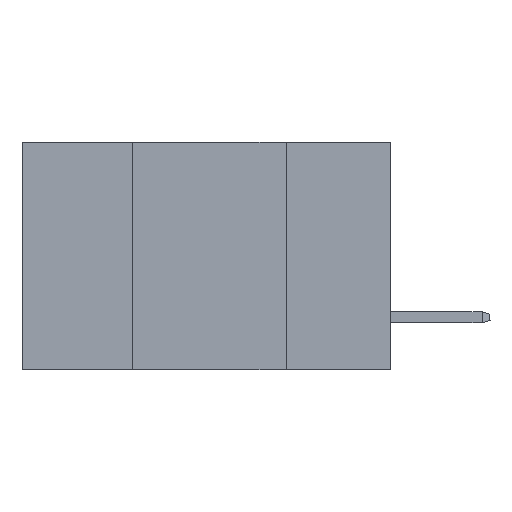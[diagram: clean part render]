
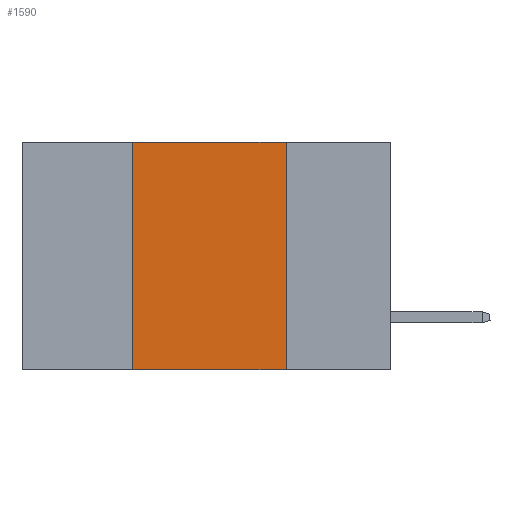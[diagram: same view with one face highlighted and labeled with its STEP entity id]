
A CAD part, left-side view. The second image highlights one B-rep face of the part: STEP entity #1590.
In plain terms, the highlighted planar face has unit normal (-1, 0, 0).
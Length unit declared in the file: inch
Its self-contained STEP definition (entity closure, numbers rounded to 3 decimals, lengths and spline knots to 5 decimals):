
#1293 = CARTESIAN_POINT ( 'NONE',  ( 0., 0.17, 0. ) ) ;
#1590 = ADVANCED_FACE ( 'NONE', ( #4072 ), #20724, .F. ) ;
#1741 = ORIENTED_EDGE ( 'NONE', *, *, #5785, .T. ) ;
#2574 = CARTESIAN_POINT ( 'NONE',  ( 0., 0.42, -0.37 ) ) ;
#3450 = CARTESIAN_POINT ( 'NONE',  ( 0., 0.6, 0. ) ) ;
#4072 = FACE_OUTER_BOUND ( 'NONE', #17372, .T. ) ;
#4275 = ORIENTED_EDGE ( 'NONE', *, *, #7892, .F. ) ;
#4960 = CARTESIAN_POINT ( 'NONE',  ( 0., 0.42, 0. ) ) ;
#5785 = EDGE_CURVE ( 'NONE', #17958, #6921, #11156, .T. ) ;
#6727 = VERTEX_POINT ( 'NONE', #1293 ) ;
#6910 = VECTOR ( 'NONE', #20247, 39.37008 ) ;
#6921 = VERTEX_POINT ( 'NONE', #15824 ) ;
#7892 = EDGE_CURVE ( 'NONE', #19741, #6727, #8213, .T. ) ;
#8213 = LINE ( 'NONE', #24294, #20574 ) ;
#9295 = DIRECTION ( 'NONE',  ( 0., 0., -1. ) ) ;
#11156 = LINE ( 'NONE', #16018, #18658 ) ;
#11177 = CARTESIAN_POINT ( 'NONE',  ( 0., 0.17, 0. ) ) ;
#12067 = LINE ( 'NONE', #4960, #6910 ) ;
#14723 = DIRECTION ( 'NONE',  ( 1., 0., 0. ) ) ;
#15048 = DIRECTION ( 'NONE',  ( 0., 0., -1. ) ) ;
#15365 = EDGE_CURVE ( 'NONE', #17958, #19741, #12067, .T. ) ;
#15824 = CARTESIAN_POINT ( 'NONE',  ( 0., 0.17, -0.37 ) ) ;
#16018 = CARTESIAN_POINT ( 'NONE',  ( 0., 0.6, -0.37 ) ) ;
#16765 = DIRECTION ( 'NONE',  ( 0., -1., 0. ) ) ;
#17372 = EDGE_LOOP ( 'NONE', ( #19677, #4275, #23735, #1741 ) ) ;
#17938 = DIRECTION ( 'NONE',  ( 0., -1., 0. ) ) ;
#17958 = VERTEX_POINT ( 'NONE', #2574 ) ;
#17992 = VECTOR ( 'NONE', #15048, 39.37008 ) ;
#18658 = VECTOR ( 'NONE', #17938, 39.37008 ) ;
#18881 = LINE ( 'NONE', #11177, #17992 ) ;
#19083 = AXIS2_PLACEMENT_3D ( 'NONE', #3450, #14723, #9295 ) ;
#19677 = ORIENTED_EDGE ( 'NONE', *, *, #24018, .F. ) ;
#19741 = VERTEX_POINT ( 'NONE', #21061 ) ;
#20247 = DIRECTION ( 'NONE',  ( 0., 0., 1. ) ) ;
#20574 = VECTOR ( 'NONE', #16765, 39.37008 ) ;
#20724 = PLANE ( 'NONE',  #19083 ) ;
#21061 = CARTESIAN_POINT ( 'NONE',  ( 0., 0.42, 0. ) ) ;
#23735 = ORIENTED_EDGE ( 'NONE', *, *, #15365, .F. ) ;
#24018 = EDGE_CURVE ( 'NONE', #6727, #6921, #18881, .T. ) ;
#24294 = CARTESIAN_POINT ( 'NONE',  ( 0., 0.6, 0. ) ) ;
